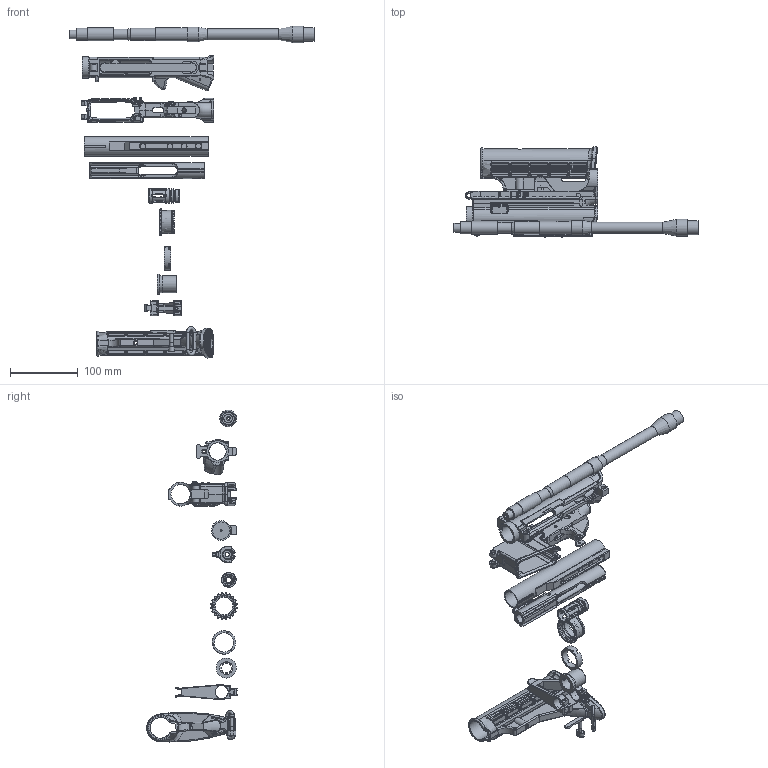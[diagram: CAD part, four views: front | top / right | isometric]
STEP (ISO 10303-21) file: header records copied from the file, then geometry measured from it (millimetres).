
FILE_DESCRIPTION (( 'STEP AP214' ), '1' );
FILE_NAME ('Unthreaded Components.STEP', '2019-03-20T16:32:43', ( 'Windows-Benutzer' ), ( '' ), 'SwSTEP 2.0', 'SolidWorks 2018', '' );
FILE_SCHEMA (( 'AUTOMOTIVE_DESIGN' ));
Length unit declared in the file: millimetre
Products named in the file (18): Front Sight Post.step; Stock Body.step; Stock Swivel.step; Upper Receiver Body.step; Bolt Carrier Gas Key.step; Flash Hider.step; Magazine Catch Button.step; Castle Nut.step; Barrel Extension.step; Bolt Carrier.step; Unthreaded Components; Magazine Catch Bar.step; Buffer Tube Body.step; Barrel Nut.step; Lower Receiver Body.step; Front Sight.step; Unthreaded Components.step; Barrel.step
Assembly tree (17 placements, depth 3):
  Unthreaded Components
    Unthreaded Components.step
      Barrel.step
      Upper Receiver Body.step
      Lower Receiver Body.step
      Buffer Tube Body.step
      Castle Nut.step
      Barrel Extension.step
      Barrel Nut.step
      Flash Hider.step
      Front Sight Post.step
      Magazine Catch Bar.step
      Magazine Catch Button.step
      Bolt Carrier.step
      Bolt Carrier Gas Key.step
      Stock Swivel.step
      Stock Body.step
      Front Sight.step
Bounding box: 360.58 x 133.79 x 490.52 mm (x, y, z)
Volume: 461208.6 mm3; surface area: 290408.1 mm2
Topology: 16 solids, 16 shells, 6777 faces, 17755 edges, 11504 vertices
Faces by surface type: plane 4029, bspline 1189, cylinder 1000, torus 326, cone 172, sphere 61
Full cylindrical faces by diameter (mm): 1.981 x3, 2.286 x2, 2.388 x2, 2.4 x2, 2.464 x4, 2.794 x2, 2.87 x1, 3.175 x4, 3.2 x1, 3.239 x2, 3.277 x2, 3.454 x3, 3.581 x2, 3.683 x2, 3.95 x1, 3.962 x5, 4.039 x1, 4.064 x1, 4.293 x1, 4.343 x1, 4.366 x1, 4.369 x2, 4.585 x2, 4.623 x1, 4.648 x1, 4.712 x1, 4.75 x1, 4.933 x1, 5.2 x1, 5.55 x1
Entity records: 344610 total; most frequent: CARTESIAN_POINT 205285, ORIENTED_EDGE 34824, DIRECTION 18288, EDGE_CURVE 17412, B_SPLINE_CURVE_WITH_KNOTS 11898, VERTEX_POINT 11403, EDGE_LOOP 7685, AXIS2_PLACEMENT_3D 7463
